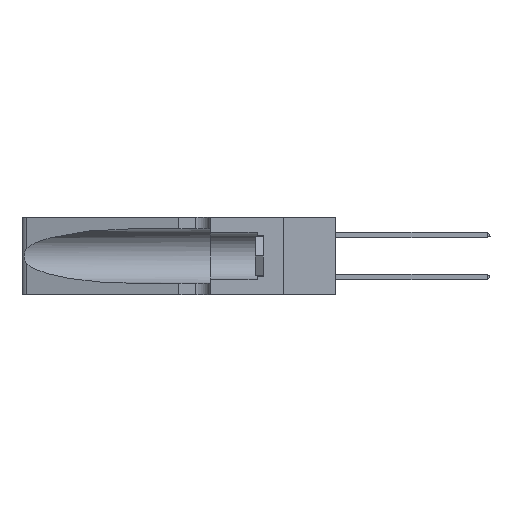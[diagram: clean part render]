
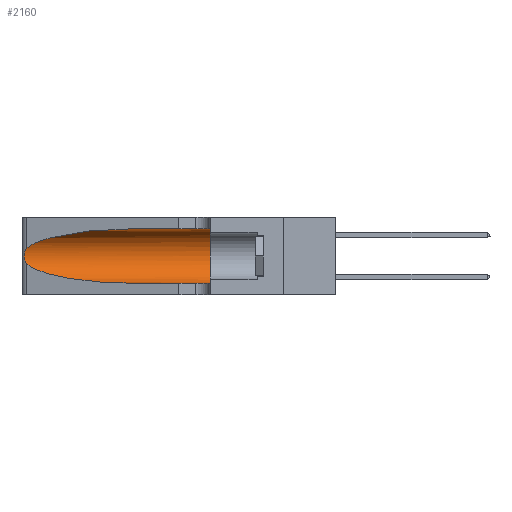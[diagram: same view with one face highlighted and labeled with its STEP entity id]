
A CAD part, left-side view. The second image highlights one B-rep face of the part: STEP entity #2160.
In plain terms, the highlighted cylindrical face has radius 3.308 mm (diameter 6.617 mm), a partial arc.
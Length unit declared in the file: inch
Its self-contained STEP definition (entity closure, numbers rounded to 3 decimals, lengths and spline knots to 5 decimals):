
#635 = CARTESIAN_POINT ( 'NONE',  ( 0.1305, 0.72297, 0.05475 ) ) ;
#1766 = CARTESIAN_POINT ( 'NONE',  ( 0.25787, 1.23484, 0.2124 ) ) ;
#2117 = VERTEX_POINT ( 'NONE', #29537 ) ;
#2160 = ADVANCED_FACE ( 'NONE', ( #13118 ), #37096, .F. ) ;
#2839 = DIRECTION ( 'NONE',  ( 0., -1., 0. ) ) ;
#2989 = CARTESIAN_POINT ( 'NONE',  ( 0.1305, 0.35, 0.31525 ) ) ;
#3208 = LINE ( 'NONE', #43732, #39509 ) ;
#4699 = EDGE_CURVE ( 'NONE', #25008, #2117, #31848, .T. ) ;
#4996 = VERTEX_POINT ( 'NONE', #40747 ) ;
#5037 = CARTESIAN_POINT ( 'NONE',  ( 0.1305, 0.72297, 0.05475 ) ) ;
#5243 = CARTESIAN_POINT ( 'NONE',  ( 0.26018, 1.23835, 0.19895 ) ) ;
#5892 = EDGE_LOOP ( 'NONE', ( #15428, #14723, #12745, #33947, #11135, #13363 ) ) ;
#8778 = CARTESIAN_POINT ( 'NONE',  ( 0.26075, 1.23896, 0.178 ) ) ;
#9266 = CARTESIAN_POINT ( 'NONE',  ( 0.1305, 1.61858, 0.185 ) ) ;
#9268 = CIRCLE ( 'NONE', #25456, 0.13025 ) ;
#11135 = ORIENTED_EDGE ( 'NONE', *, *, #30267, .F. ) ;
#12043 = CARTESIAN_POINT ( 'NONE',  ( 0.25555, 1.22994, 0.2215 ) ) ;
#12129 =( BOUNDED_CURVE ( )  B_SPLINE_CURVE ( 3, ( #30239, #33681, #16685, #40455 ),
 .UNSPECIFIED., .F., .T. ) 
 B_SPLINE_CURVE_WITH_KNOTS ( ( 4, 4 ),
 ( 1.5708, 2.84003 ),
 .UNSPECIFIED. ) 
 CURVE ( )  GEOMETRIC_REPRESENTATION_ITEM ( )  RATIONAL_B_SPLINE_CURVE ( ( 1., 0.87, 0.87, 1. ) ) 
 REPRESENTATION_ITEM ( '' )  );
#12199 = CARTESIAN_POINT ( 'NONE',  ( 0.25856, 1.23593, 0.16098 ) ) ;
#12745 = ORIENTED_EDGE ( 'NONE', *, *, #16565, .T. ) ;
#13118 = FACE_OUTER_BOUND ( 'NONE', #5892, .T. ) ;
#13363 = ORIENTED_EDGE ( 'NONE', *, *, #16119, .F. ) ;
#14697 = CARTESIAN_POINT ( 'NONE',  ( 0.1305, 0.35, 0.185 ) ) ;
#14723 = ORIENTED_EDGE ( 'NONE', *, *, #4699, .T. ) ;
#15387 = VERTEX_POINT ( 'NONE', #36835 ) ;
#15428 = ORIENTED_EDGE ( 'NONE', *, *, #28250, .T. ) ;
#15614 = CARTESIAN_POINT ( 'NONE',  ( 0.25639, 1.23186, 0.15144 ) ) ;
#15745 = VECTOR ( 'NONE', #26482, 39.37008 ) ;
#16119 = EDGE_CURVE ( 'NONE', #4996, #38944, #3208, .T. ) ;
#16565 = EDGE_CURVE ( 'NONE', #2117, #34658, #24502, .T. ) ;
#16685 = CARTESIAN_POINT ( 'NONE',  ( 0.2373, 1.15595, 0.28018 ) ) ;
#18140 = DIRECTION ( 'NONE',  ( 0., 0., 1. ) ) ;
#19082 = CARTESIAN_POINT ( 'NONE',  ( 0.25487, 1.22718, 0.14631 ) ) ;
#22157 = CARTESIAN_POINT ( 'NONE',  ( 0.2373, 1.15595, 0.08982 ) ) ;
#22352 = CARTESIAN_POINT ( 'NONE',  ( 0.25639, 1.23184, 0.21858 ) ) ;
#23055 = CARTESIAN_POINT ( 'NONE',  ( 0.1305, 1.61858, 0.05475 ) ) ;
#24502 =( BOUNDED_CURVE ( )  B_SPLINE_CURVE ( 3, ( #32274, #22157, #25566, #5037 ),
 .UNSPECIFIED., .F., .F. ) 
 B_SPLINE_CURVE_WITH_KNOTS ( ( 4, 4 ),
 ( 3.44316, 4.71239 ),
 .UNSPECIFIED. ) 
 CURVE ( )  GEOMETRIC_REPRESENTATION_ITEM ( )  RATIONAL_B_SPLINE_CURVE ( ( 1., 0.87, 0.87, 1. ) ) 
 REPRESENTATION_ITEM ( '' )  );
#25008 = VERTEX_POINT ( 'NONE', #35957 ) ;
#25456 = AXIS2_PLACEMENT_3D ( 'NONE', #14697, #38494, #18140 ) ;
#25566 = CARTESIAN_POINT ( 'NONE',  ( 0.18966, 0.96281, 0.05475 ) ) ;
#25774 = CARTESIAN_POINT ( 'NONE',  ( 0.25854, 1.2359, 0.20912 ) ) ;
#26482 = DIRECTION ( 'NONE',  ( 0., -1., 0. ) ) ;
#28250 = EDGE_CURVE ( 'NONE', #4996, #25008, #12129, .T. ) ;
#28729 = EDGE_CURVE ( 'NONE', #34658, #15387, #33927, .T. ) ;
#28916 = CARTESIAN_POINT ( 'NONE',  ( 0.25487, 1.22718, 0.22369 ) ) ;
#29197 = CARTESIAN_POINT ( 'NONE',  ( 0.26075, 1.23896, 0.19203 ) ) ;
#29537 = CARTESIAN_POINT ( 'NONE',  ( 0.25487, 1.22718, 0.14631 ) ) ;
#29687 = DIRECTION ( 'NONE',  ( 0., 0., -1. ) ) ;
#30239 = CARTESIAN_POINT ( 'NONE',  ( 0.1305, 0.72297, 0.31525 ) ) ;
#30267 = EDGE_CURVE ( 'NONE', #38944, #15387, #9268, .T. ) ;
#31848 = B_SPLINE_CURVE_WITH_KNOTS ( 'NONE', 3,
 ( #28916, #12043, #22352, #1766, #25774, #5243, #29197, #8778, #32620, #12199, #36046, #15614, #39420, #19082 ),
 .UNSPECIFIED., .F., .F.,
 ( 4, 2, 2, 2, 2, 2, 4 ),
 ( 0., 0.00027, 0.00053, 0.00107, 0.0016, 0.00187, 0.00214 ),
 .UNSPECIFIED. ) ;
#32274 = CARTESIAN_POINT ( 'NONE',  ( 0.25487, 1.22718, 0.14631 ) ) ;
#32620 = CARTESIAN_POINT ( 'NONE',  ( 0.26017, 1.23833, 0.17102 ) ) ;
#33681 = CARTESIAN_POINT ( 'NONE',  ( 0.18966, 0.96281, 0.31525 ) ) ;
#33927 = LINE ( 'NONE', #23055, #15745 ) ;
#33947 = ORIENTED_EDGE ( 'NONE', *, *, #28729, .T. ) ;
#34658 = VERTEX_POINT ( 'NONE', #635 ) ;
#35742 = AXIS2_PLACEMENT_3D ( 'NONE', #9266, #43334, #29687 ) ;
#35957 = CARTESIAN_POINT ( 'NONE',  ( 0.25487, 1.22718, 0.22369 ) ) ;
#36046 = CARTESIAN_POINT ( 'NONE',  ( 0.25789, 1.23486, 0.15765 ) ) ;
#36835 = CARTESIAN_POINT ( 'NONE',  ( 0.1305, 0.35, 0.05475 ) ) ;
#37096 = CYLINDRICAL_SURFACE ( 'NONE', #35742, 0.13025 ) ;
#38494 = DIRECTION ( 'NONE',  ( 0., 1., 0. ) ) ;
#38944 = VERTEX_POINT ( 'NONE', #2989 ) ;
#39420 = CARTESIAN_POINT ( 'NONE',  ( 0.25555, 1.22993, 0.14849 ) ) ;
#39509 = VECTOR ( 'NONE', #2839, 39.37008 ) ;
#40455 = CARTESIAN_POINT ( 'NONE',  ( 0.25487, 1.22718, 0.22369 ) ) ;
#40747 = CARTESIAN_POINT ( 'NONE',  ( 0.1305, 0.72297, 0.31525 ) ) ;
#43334 = DIRECTION ( 'NONE',  ( 0., -1., 0. ) ) ;
#43732 = CARTESIAN_POINT ( 'NONE',  ( 0.1305, 1.61858, 0.31525 ) ) ;
